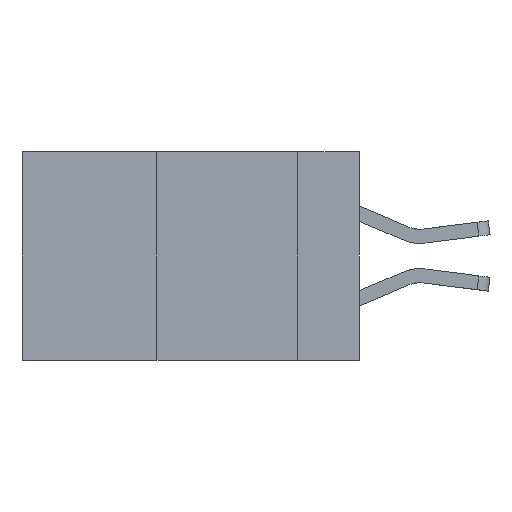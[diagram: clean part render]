
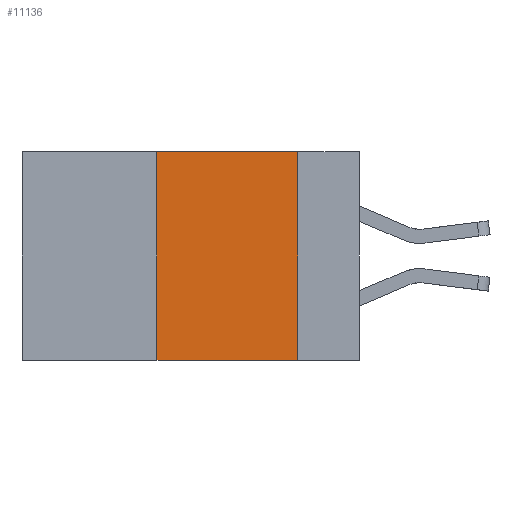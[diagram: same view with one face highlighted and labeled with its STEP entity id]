
A CAD part, left-side view. The second image highlights one B-rep face of the part: STEP entity #11136.
In plain terms, the highlighted planar face has unit normal (-1, 0, 0).
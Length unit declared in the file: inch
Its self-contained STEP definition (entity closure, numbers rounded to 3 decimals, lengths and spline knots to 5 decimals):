
#678 = VERTEX_POINT ( 'NONE', #7728 ) ;
#1207 = DIRECTION ( 'NONE',  ( 1., 0., 0. ) ) ;
#1281 = EDGE_CURVE ( 'NONE', #11850, #2275, #9983, .T. ) ;
#1581 = VECTOR ( 'NONE', #10369, 39.37008 ) ;
#1611 = EDGE_LOOP ( 'NONE', ( #7266, #2614, #6853, #7318 ) ) ;
#1943 = VERTEX_POINT ( 'NONE', #4205 ) ;
#2275 = VERTEX_POINT ( 'NONE', #11856 ) ;
#2614 = ORIENTED_EDGE ( 'NONE', *, *, #11641, .F. ) ;
#4035 = LINE ( 'NONE', #5025, #11351 ) ;
#4205 = CARTESIAN_POINT ( 'NONE',  ( 0., 0.11, 0. ) ) ;
#4371 = CARTESIAN_POINT ( 'NONE',  ( 0., 0.36, -0.37 ) ) ;
#5009 = EDGE_CURVE ( 'NONE', #11850, #678, #4035, .T. ) ;
#5025 = CARTESIAN_POINT ( 'NONE',  ( 0., 0.36, 0. ) ) ;
#5527 = AXIS2_PLACEMENT_3D ( 'NONE', #7099, #1207, #8105 ) ;
#5529 = LINE ( 'NONE', #8464, #7456 ) ;
#5776 = LINE ( 'NONE', #6921, #10534 ) ;
#6677 = EDGE_CURVE ( 'NONE', #1943, #2275, #5529, .T. ) ;
#6853 = ORIENTED_EDGE ( 'NONE', *, *, #5009, .F. ) ;
#6921 = CARTESIAN_POINT ( 'NONE',  ( 0., 0.6, 0. ) ) ;
#7099 = CARTESIAN_POINT ( 'NONE',  ( 0., 0.6, 0. ) ) ;
#7266 = ORIENTED_EDGE ( 'NONE', *, *, #6677, .F. ) ;
#7318 = ORIENTED_EDGE ( 'NONE', *, *, #1281, .T. ) ;
#7456 = VECTOR ( 'NONE', #11286, 39.37008 ) ;
#7728 = CARTESIAN_POINT ( 'NONE',  ( 0., 0.36, 0. ) ) ;
#7916 = DIRECTION ( 'NONE',  ( 0., -1., 0. ) ) ;
#8105 = DIRECTION ( 'NONE',  ( 0., 0., -1. ) ) ;
#8464 = CARTESIAN_POINT ( 'NONE',  ( 0., 0.11, 0. ) ) ;
#9256 = FACE_OUTER_BOUND ( 'NONE', #1611, .T. ) ;
#9983 = LINE ( 'NONE', #10185, #1581 ) ;
#10185 = CARTESIAN_POINT ( 'NONE',  ( 0., 0.6, -0.37 ) ) ;
#10369 = DIRECTION ( 'NONE',  ( 0., -1., 0. ) ) ;
#10534 = VECTOR ( 'NONE', #7916, 39.37008 ) ;
#11136 = ADVANCED_FACE ( 'NONE', ( #9256 ), #11808, .F. ) ;
#11286 = DIRECTION ( 'NONE',  ( 0., 0., -1. ) ) ;
#11351 = VECTOR ( 'NONE', #11669, 39.37008 ) ;
#11641 = EDGE_CURVE ( 'NONE', #678, #1943, #5776, .T. ) ;
#11669 = DIRECTION ( 'NONE',  ( 0., 0., 1. ) ) ;
#11808 = PLANE ( 'NONE',  #5527 ) ;
#11850 = VERTEX_POINT ( 'NONE', #4371 ) ;
#11856 = CARTESIAN_POINT ( 'NONE',  ( 0., 0.11, -0.37 ) ) ;
